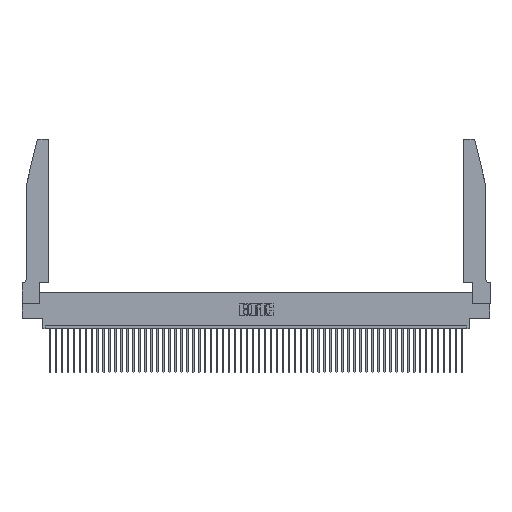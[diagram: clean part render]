
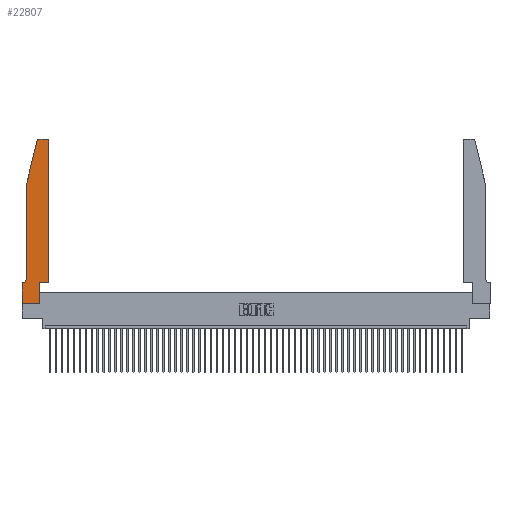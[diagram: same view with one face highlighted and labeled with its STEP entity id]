
A CAD part, top view. The second image highlights one B-rep face of the part: STEP entity #22807.
In plain terms, the highlighted planar face has unit normal (0, 0, 1).
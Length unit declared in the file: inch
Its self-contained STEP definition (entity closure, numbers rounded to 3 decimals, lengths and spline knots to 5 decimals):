
#26 = VECTOR ( 'NONE', #43180, 39.37008 ) ;
#43 = EDGE_CURVE ( 'NONE', #34394, #7416, #30765, .T. ) ;
#242 = EDGE_CURVE ( 'NONE', #9578, #16684, #1462, .T. ) ;
#867 = CARTESIAN_POINT ( 'NONE',  ( 0.0055, 0.35, 0.37 ) ) ;
#1121 = VECTOR ( 'NONE', #43523, 39.37008 ) ;
#1462 = LINE ( 'NONE', #17534, #22854 ) ;
#2064 = VERTEX_POINT ( 'NONE', #867 ) ;
#2176 = VECTOR ( 'NONE', #40880, 39.37008 ) ;
#2520 = CIRCLE ( 'NONE', #5980, 0.03 ) ;
#2804 = DIRECTION ( 'NONE',  ( 1., 0., 0. ) ) ;
#2810 = ORIENTED_EDGE ( 'NONE', *, *, #4100, .T. ) ;
#2926 = ORIENTED_EDGE ( 'NONE', *, *, #7846, .T. ) ;
#3640 = CIRCLE ( 'NONE', #46406, 0.03 ) ;
#3644 = VERTEX_POINT ( 'NONE', #32552 ) ;
#3777 = LINE ( 'NONE', #14251, #1121 ) ;
#4100 = EDGE_CURVE ( 'NONE', #16566, #23244, #28193, .T. ) ;
#4808 = CIRCLE ( 'NONE', #19740, 0.07 ) ;
#5749 = CARTESIAN_POINT ( 'NONE',  ( 0.4205, 2.72, 0.37 ) ) ;
#5847 = CARTESIAN_POINT ( 'NONE',  ( 0., 0.35, 0.37 ) ) ;
#5980 = AXIS2_PLACEMENT_3D ( 'NONE', #21424, #25268, #25794 ) ;
#6122 = CARTESIAN_POINT ( 'NONE',  ( 0.4205, 2.75, 0.37 ) ) ;
#6514 = CARTESIAN_POINT ( 'NONE',  ( 0.4505, 0.35, 0.37 ) ) ;
#7416 = VERTEX_POINT ( 'NONE', #38004 ) ;
#7846 = EDGE_CURVE ( 'NONE', #13304, #40336, #47304, .T. ) ;
#8532 = LINE ( 'NONE', #29045, #35892 ) ;
#8882 = AXIS2_PLACEMENT_3D ( 'NONE', #14556, #31663, #2804 ) ;
#9578 = VERTEX_POINT ( 'NONE', #6514 ) ;
#9882 = DIRECTION ( 'NONE',  ( 0., 0., 1. ) ) ;
#10260 = CARTESIAN_POINT ( 'NONE',  ( 0.0055, 0.42, 0.37 ) ) ;
#12535 = DIRECTION ( 'NONE',  ( 0., -1., 0. ) ) ;
#13304 = VERTEX_POINT ( 'NONE', #19766 ) ;
#14027 = ORIENTED_EDGE ( 'NONE', *, *, #43, .T. ) ;
#14251 = CARTESIAN_POINT ( 'NONE',  ( 0.0755, 0.35, 0.37 ) ) ;
#14543 = EDGE_CURVE ( 'NONE', #23244, #13304, #51375, .T. ) ;
#14556 = CARTESIAN_POINT ( 'NONE',  ( 0., 0.35, 0.37 ) ) ;
#15724 = VERTEX_POINT ( 'NONE', #39324 ) ;
#16566 = VERTEX_POINT ( 'NONE', #5847 ) ;
#16684 = VERTEX_POINT ( 'NONE', #19455 ) ;
#17382 = ORIENTED_EDGE ( 'NONE', *, *, #45420, .T. ) ;
#17534 = CARTESIAN_POINT ( 'NONE',  ( 0.4505, 0.35, 0.37 ) ) ;
#18746 = CARTESIAN_POINT ( 'NONE',  ( 0., 0., 0.37 ) ) ;
#18866 = ORIENTED_EDGE ( 'NONE', *, *, #44142, .T. ) ;
#19240 = EDGE_CURVE ( 'NONE', #16684, #34394, #3640, .T. ) ;
#19455 = CARTESIAN_POINT ( 'NONE',  ( 0.4505, 2.72, 0.37 ) ) ;
#19740 = AXIS2_PLACEMENT_3D ( 'NONE', #10260, #40632, #43892 ) ;
#19766 = CARTESIAN_POINT ( 'NONE',  ( 0.2865, 0., 0.37 ) ) ;
#19935 = DIRECTION ( 'NONE',  ( 1., 0., 0. ) ) ;
#20773 = LINE ( 'NONE', #47385, #26 ) ;
#20845 = VECTOR ( 'NONE', #47537, 39.37008 ) ;
#21028 = DIRECTION ( 'NONE',  ( 0., -1., 0. ) ) ;
#21424 = CARTESIAN_POINT ( 'NONE',  ( 0.284, 2.72, 0.37 ) ) ;
#21489 = ORIENTED_EDGE ( 'NONE', *, *, #19240, .T. ) ;
#22267 = CARTESIAN_POINT ( 'NONE',  ( 0.0755, 0.42, 0.37 ) ) ;
#22807 = ADVANCED_FACE ( 'NONE', ( #46162 ), #23462, .T. ) ;
#22854 = VECTOR ( 'NONE', #29896, 39.37008 ) ;
#23244 = VERTEX_POINT ( 'NONE', #18746 ) ;
#23462 = PLANE ( 'NONE',  #8882 ) ;
#23960 = CARTESIAN_POINT ( 'NONE',  ( 0.2605, 2.75, 0.37 ) ) ;
#24953 = VECTOR ( 'NONE', #12535, 39.37008 ) ;
#25268 = DIRECTION ( 'NONE',  ( 0., 0., 1. ) ) ;
#25794 = DIRECTION ( 'NONE',  ( 1., 0., 0. ) ) ;
#25997 = ORIENTED_EDGE ( 'NONE', *, *, #30213, .T. ) ;
#26953 = DIRECTION ( 'NONE',  ( 1., 0., 0. ) ) ;
#27264 = CARTESIAN_POINT ( 'NONE',  ( 0.2865, 0.35, 0.37 ) ) ;
#27707 = DIRECTION ( 'NONE',  ( 0., 1., 0. ) ) ;
#28193 = LINE ( 'NONE', #49742, #24953 ) ;
#28512 = ORIENTED_EDGE ( 'NONE', *, *, #34322, .T. ) ;
#29045 = CARTESIAN_POINT ( 'NONE',  ( 0.0755, 2., 0.37 ) ) ;
#29896 = DIRECTION ( 'NONE',  ( 0., 1., 0. ) ) ;
#30213 = EDGE_CURVE ( 'NONE', #3644, #15724, #20773, .T. ) ;
#30440 = EDGE_LOOP ( 'NONE', ( #14027, #38316, #25997, #36439, #18866, #28512, #2810, #32794, #2926, #17382, #40010, #21489 ) ) ;
#30765 = LINE ( 'NONE', #23960, #2176 ) ;
#31367 = CARTESIAN_POINT ( 'NONE',  ( 0.2865, 0.35, 0.37 ) ) ;
#31663 = DIRECTION ( 'NONE',  ( 0., 0., 1. ) ) ;
#32552 = CARTESIAN_POINT ( 'NONE',  ( 0.25487, 2.72718, 0.37 ) ) ;
#32794 = ORIENTED_EDGE ( 'NONE', *, *, #14543, .T. ) ;
#34322 = EDGE_CURVE ( 'NONE', #2064, #16566, #3777, .T. ) ;
#34394 = VERTEX_POINT ( 'NONE', #6122 ) ;
#35892 = VECTOR ( 'NONE', #21028, 39.37008 ) ;
#36332 = VERTEX_POINT ( 'NONE', #22267 ) ;
#36439 = ORIENTED_EDGE ( 'NONE', *, *, #48167, .T. ) ;
#38004 = CARTESIAN_POINT ( 'NONE',  ( 0.284, 2.75, 0.37 ) ) ;
#38316 = ORIENTED_EDGE ( 'NONE', *, *, #40877, .T. ) ;
#39324 = CARTESIAN_POINT ( 'NONE',  ( 0.0755, 2., 0.37 ) ) ;
#40010 = ORIENTED_EDGE ( 'NONE', *, *, #242, .T. ) ;
#40336 = VERTEX_POINT ( 'NONE', #27264 ) ;
#40632 = DIRECTION ( 'NONE',  ( 0., 0., -1. ) ) ;
#40877 = EDGE_CURVE ( 'NONE', #7416, #3644, #2520, .T. ) ;
#40880 = DIRECTION ( 'NONE',  ( -1., 0., 0. ) ) ;
#41032 = CARTESIAN_POINT ( 'NONE',  ( 0.4505, 0.35, 0.37 ) ) ;
#41720 = VECTOR ( 'NONE', #19935, 39.37008 ) ;
#43180 = DIRECTION ( 'NONE',  ( -0.239, -0.971, 0. ) ) ;
#43336 = CARTESIAN_POINT ( 'NONE',  ( 0., 0., 0.37 ) ) ;
#43523 = DIRECTION ( 'NONE',  ( -1., 0., 0. ) ) ;
#43892 = DIRECTION ( 'NONE',  ( -1., 0., 0. ) ) ;
#44142 = EDGE_CURVE ( 'NONE', #36332, #2064, #4808, .T. ) ;
#45420 = EDGE_CURVE ( 'NONE', #40336, #9578, #52769, .T. ) ;
#46162 = FACE_OUTER_BOUND ( 'NONE', #30440, .T. ) ;
#46406 = AXIS2_PLACEMENT_3D ( 'NONE', #5749, #9882, #26953 ) ;
#47304 = LINE ( 'NONE', #31367, #53146 ) ;
#47385 = CARTESIAN_POINT ( 'NONE',  ( 0.0755, 2., 0.37 ) ) ;
#47537 = DIRECTION ( 'NONE',  ( 1., 0., 0. ) ) ;
#48167 = EDGE_CURVE ( 'NONE', #15724, #36332, #8532, .T. ) ;
#49742 = CARTESIAN_POINT ( 'NONE',  ( 0., 0., 0.37 ) ) ;
#51375 = LINE ( 'NONE', #43336, #20845 ) ;
#52769 = LINE ( 'NONE', #41032, #41720 ) ;
#53146 = VECTOR ( 'NONE', #27707, 39.37008 ) ;
